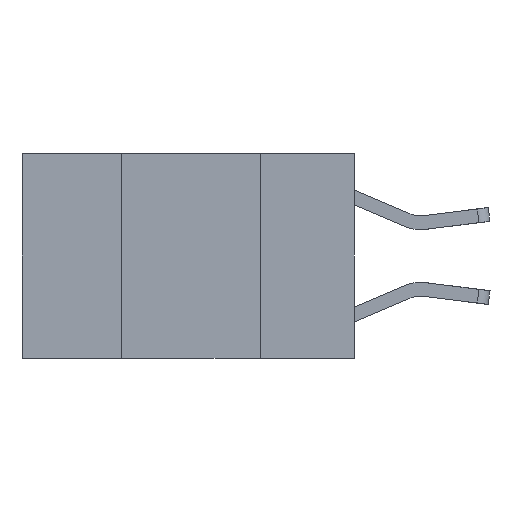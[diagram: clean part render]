
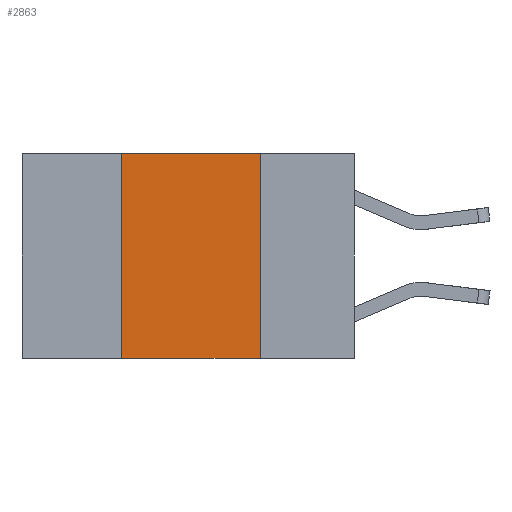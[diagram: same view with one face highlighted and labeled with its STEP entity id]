
A CAD part, left-side view. The second image highlights one B-rep face of the part: STEP entity #2863.
In plain terms, the highlighted planar face has unit normal (-1, 0, 0).
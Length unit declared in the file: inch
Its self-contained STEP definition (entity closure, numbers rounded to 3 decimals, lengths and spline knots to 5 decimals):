
#8 = DIRECTION ( 'NONE',  ( 0., -1., 0. ) ) ;
#577 = CARTESIAN_POINT ( 'NONE',  ( 0., 0.17, 0. ) ) ;
#1112 = EDGE_CURVE ( 'NONE', #4147, #8307, #4819, .T. ) ;
#1569 = ORIENTED_EDGE ( 'NONE', *, *, #6040, .T. ) ;
#1843 = ORIENTED_EDGE ( 'NONE', *, *, #1112, .F. ) ;
#2016 = DIRECTION ( 'NONE',  ( 0., 0., -1. ) ) ;
#2227 = CARTESIAN_POINT ( 'NONE',  ( 0., 0.42, -0.37 ) ) ;
#2306 = CARTESIAN_POINT ( 'NONE',  ( 0., 0.17, -0.37 ) ) ;
#2863 = ADVANCED_FACE ( 'NONE', ( #7753 ), #5941, .F. ) ;
#2916 = VERTEX_POINT ( 'NONE', #577 ) ;
#3233 = EDGE_CURVE ( 'NONE', #8307, #2916, #9282, .T. ) ;
#3506 = AXIS2_PLACEMENT_3D ( 'NONE', #5204, #8127, #3750 ) ;
#3551 = CARTESIAN_POINT ( 'NONE',  ( 0., 0.42, 0. ) ) ;
#3750 = DIRECTION ( 'NONE',  ( 0., 0., -1. ) ) ;
#4147 = VERTEX_POINT ( 'NONE', #2227 ) ;
#4450 = CARTESIAN_POINT ( 'NONE',  ( 0., 0.6, -0.37 ) ) ;
#4760 = CARTESIAN_POINT ( 'NONE',  ( 0., 0.6, 0. ) ) ;
#4814 = ORIENTED_EDGE ( 'NONE', *, *, #3233, .F. ) ;
#4819 = LINE ( 'NONE', #3551, #8658 ) ;
#5096 = CARTESIAN_POINT ( 'NONE',  ( 0., 0.42, 0. ) ) ;
#5196 = CARTESIAN_POINT ( 'NONE',  ( 0., 0.17, 0. ) ) ;
#5204 = CARTESIAN_POINT ( 'NONE',  ( 0., 0.6, 0. ) ) ;
#5479 = VECTOR ( 'NONE', #2016, 39.37008 ) ;
#5526 = VERTEX_POINT ( 'NONE', #2306 ) ;
#5929 = VECTOR ( 'NONE', #8, 39.37008 ) ;
#5941 = PLANE ( 'NONE',  #3506 ) ;
#6029 = ORIENTED_EDGE ( 'NONE', *, *, #6035, .F. ) ;
#6035 = EDGE_CURVE ( 'NONE', #2916, #5526, #7387, .T. ) ;
#6040 = EDGE_CURVE ( 'NONE', #4147, #5526, #7866, .T. ) ;
#7387 = LINE ( 'NONE', #5196, #5479 ) ;
#7753 = FACE_OUTER_BOUND ( 'NONE', #8275, .T. ) ;
#7866 = LINE ( 'NONE', #4450, #9284 ) ;
#8117 = DIRECTION ( 'NONE',  ( 0., -1., 0. ) ) ;
#8127 = DIRECTION ( 'NONE',  ( 1., 0., 0. ) ) ;
#8275 = EDGE_LOOP ( 'NONE', ( #6029, #4814, #1843, #1569 ) ) ;
#8307 = VERTEX_POINT ( 'NONE', #5096 ) ;
#8658 = VECTOR ( 'NONE', #8774, 39.37008 ) ;
#8774 = DIRECTION ( 'NONE',  ( 0., 0., 1. ) ) ;
#9282 = LINE ( 'NONE', #4760, #5929 ) ;
#9284 = VECTOR ( 'NONE', #8117, 39.37008 ) ;
